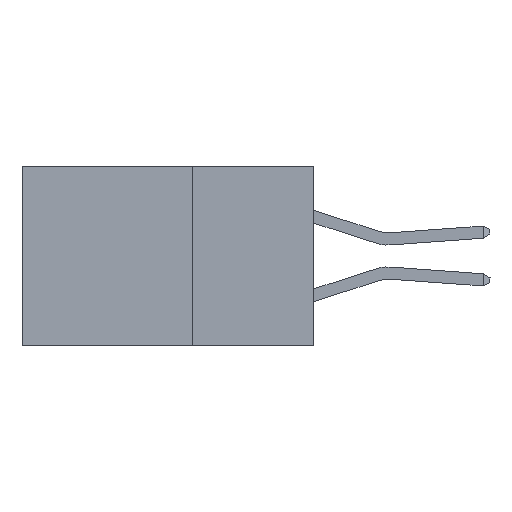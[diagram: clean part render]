
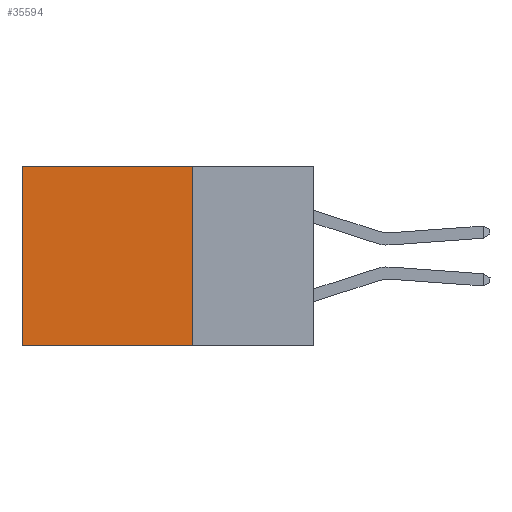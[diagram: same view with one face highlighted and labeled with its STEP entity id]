
A CAD part, left-side view. The second image highlights one B-rep face of the part: STEP entity #35594.
In plain terms, the highlighted planar face has unit normal (-1, 0, 0).
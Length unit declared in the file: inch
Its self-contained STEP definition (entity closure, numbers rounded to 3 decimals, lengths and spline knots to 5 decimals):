
#331 = EDGE_CURVE ( 'NONE', #31752, #34233, #16155, .T. ) ;
#929 = EDGE_LOOP ( 'NONE', ( #21196, #29069, #17291, #22877 ) ) ;
#1252 = DIRECTION ( 'NONE',  ( 0., 1., 0. ) ) ;
#1378 = LINE ( 'NONE', #15985, #25303 ) ;
#2914 = CARTESIAN_POINT ( 'NONE',  ( 0.2875, 0.6, 0. ) ) ;
#5591 = AXIS2_PLACEMENT_3D ( 'NONE', #35749, #10976, #38798 ) ;
#5680 = DIRECTION ( 'NONE',  ( 0., 1., 0. ) ) ;
#6728 = EDGE_CURVE ( 'NONE', #16084, #27117, #1378, .T. ) ;
#7476 = CARTESIAN_POINT ( 'NONE',  ( 0.2875, 0.25, -0.37 ) ) ;
#10976 = DIRECTION ( 'NONE',  ( 1., 0., 0. ) ) ;
#11716 = CARTESIAN_POINT ( 'NONE',  ( 0.2875, 0.25, 0. ) ) ;
#12898 = FACE_OUTER_BOUND ( 'NONE', #929, .T. ) ;
#14136 = PLANE ( 'NONE',  #5591 ) ;
#14908 = VECTOR ( 'NONE', #1252, 39.37008 ) ;
#15985 = CARTESIAN_POINT ( 'NONE',  ( 0.2875, 0.25, 0. ) ) ;
#16084 = VERTEX_POINT ( 'NONE', #34516 ) ;
#16155 = LINE ( 'NONE', #2914, #26194 ) ;
#17291 = ORIENTED_EDGE ( 'NONE', *, *, #6728, .F. ) ;
#19166 = DIRECTION ( 'NONE',  ( 0., 0., -1. ) ) ;
#19794 = LINE ( 'NONE', #11716, #38834 ) ;
#21196 = ORIENTED_EDGE ( 'NONE', *, *, #331, .T. ) ;
#22778 = CARTESIAN_POINT ( 'NONE',  ( 0.2875, 0.6, -0.37 ) ) ;
#22877 = ORIENTED_EDGE ( 'NONE', *, *, #38330, .T. ) ;
#23023 = LINE ( 'NONE', #32079, #14908 ) ;
#25303 = VECTOR ( 'NONE', #19166, 39.37008 ) ;
#25865 = EDGE_CURVE ( 'NONE', #27117, #34233, #23023, .T. ) ;
#25882 = DIRECTION ( 'NONE',  ( 0., 0., -1. ) ) ;
#26194 = VECTOR ( 'NONE', #25882, 39.37008 ) ;
#27117 = VERTEX_POINT ( 'NONE', #7476 ) ;
#29069 = ORIENTED_EDGE ( 'NONE', *, *, #25865, .F. ) ;
#31752 = VERTEX_POINT ( 'NONE', #33799 ) ;
#32079 = CARTESIAN_POINT ( 'NONE',  ( 0.2875, 0.25, -0.37 ) ) ;
#33799 = CARTESIAN_POINT ( 'NONE',  ( 0.2875, 0.6, 0. ) ) ;
#34233 = VERTEX_POINT ( 'NONE', #22778 ) ;
#34516 = CARTESIAN_POINT ( 'NONE',  ( 0.2875, 0.25, 0. ) ) ;
#35594 = ADVANCED_FACE ( 'NONE', ( #12898 ), #14136, .F. ) ;
#35749 = CARTESIAN_POINT ( 'NONE',  ( 0.2875, 0.25, 0. ) ) ;
#38330 = EDGE_CURVE ( 'NONE', #16084, #31752, #19794, .T. ) ;
#38798 = DIRECTION ( 'NONE',  ( 0., 0., -1. ) ) ;
#38834 = VECTOR ( 'NONE', #5680, 39.37008 ) ;
